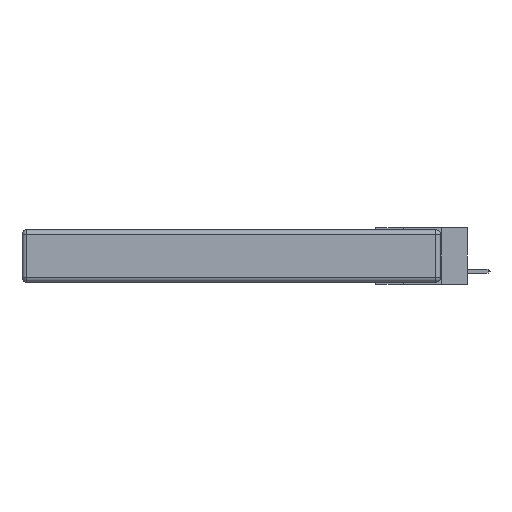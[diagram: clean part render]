
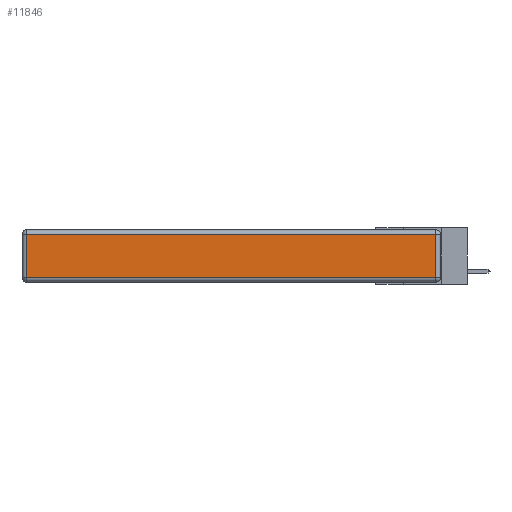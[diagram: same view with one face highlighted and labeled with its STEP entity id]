
A CAD part, left-side view. The second image highlights one B-rep face of the part: STEP entity #11846.
In plain terms, the highlighted planar face has unit normal (-1, 0, 0).
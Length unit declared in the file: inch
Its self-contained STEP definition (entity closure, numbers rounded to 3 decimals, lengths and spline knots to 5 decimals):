
#220 = EDGE_CURVE ( 'NONE', #11054, #975, #14316, .T. ) ;
#969 = AXIS2_PLACEMENT_3D ( 'NONE', #6262, #14384, #7416 ) ;
#975 = VERTEX_POINT ( 'NONE', #3014 ) ;
#1094 = EDGE_CURVE ( 'NONE', #2749, #12180, #1872, .T. ) ;
#1251 = DIRECTION ( 'NONE',  ( 0., 1., 0. ) ) ;
#1310 = CARTESIAN_POINT ( 'NONE',  ( 0., 0.03, -0.313 ) ) ;
#1872 = LINE ( 'NONE', #3119, #6068 ) ;
#2749 = VERTEX_POINT ( 'NONE', #1310 ) ;
#3014 = CARTESIAN_POINT ( 'NONE',  ( 0., 2.72, -0.313 ) ) ;
#3119 = CARTESIAN_POINT ( 'NONE',  ( 0., 0.03, -0.343 ) ) ;
#3289 = CARTESIAN_POINT ( 'NONE',  ( 0., 2.72, -0.03 ) ) ;
#3431 = CARTESIAN_POINT ( 'NONE',  ( 0., 2.75, -0.03 ) ) ;
#4220 = LINE ( 'NONE', #3431, #13159 ) ;
#4532 = EDGE_CURVE ( 'NONE', #12180, #11054, #4220, .T. ) ;
#5137 = CARTESIAN_POINT ( 'NONE',  ( 0., 0.03, -0.03 ) ) ;
#5554 = FACE_OUTER_BOUND ( 'NONE', #14267, .T. ) ;
#5933 = ORIENTED_EDGE ( 'NONE', *, *, #220, .T. ) ;
#6068 = VECTOR ( 'NONE', #11166, 39.37008 ) ;
#6146 = ORIENTED_EDGE ( 'NONE', *, *, #1094, .T. ) ;
#6213 = PLANE ( 'NONE',  #969 ) ;
#6262 = CARTESIAN_POINT ( 'NONE',  ( 0., 0., -0.343 ) ) ;
#7226 = ORIENTED_EDGE ( 'NONE', *, *, #4532, .T. ) ;
#7416 = DIRECTION ( 'NONE',  ( 0., 0., 1. ) ) ;
#7668 = LINE ( 'NONE', #11883, #12980 ) ;
#8492 = ORIENTED_EDGE ( 'NONE', *, *, #12983, .T. ) ;
#8902 = CARTESIAN_POINT ( 'NONE',  ( 0., 2.72, -0.343 ) ) ;
#9913 = DIRECTION ( 'NONE',  ( 0., 0., -1. ) ) ;
#11054 = VERTEX_POINT ( 'NONE', #3289 ) ;
#11166 = DIRECTION ( 'NONE',  ( 0., 0., 1. ) ) ;
#11846 = ADVANCED_FACE ( 'NONE', ( #5554 ), #6213, .T. ) ;
#11883 = CARTESIAN_POINT ( 'NONE',  ( 0., 0., -0.313 ) ) ;
#12180 = VERTEX_POINT ( 'NONE', #5137 ) ;
#12980 = VECTOR ( 'NONE', #13014, 39.37008 ) ;
#12983 = EDGE_CURVE ( 'NONE', #975, #2749, #7668, .T. ) ;
#13014 = DIRECTION ( 'NONE',  ( 0., -1., 0. ) ) ;
#13159 = VECTOR ( 'NONE', #1251, 39.37008 ) ;
#14267 = EDGE_LOOP ( 'NONE', ( #8492, #6146, #7226, #5933 ) ) ;
#14316 = LINE ( 'NONE', #8902, #14482 ) ;
#14384 = DIRECTION ( 'NONE',  ( -1., 0., 0. ) ) ;
#14482 = VECTOR ( 'NONE', #9913, 39.37008 ) ;
